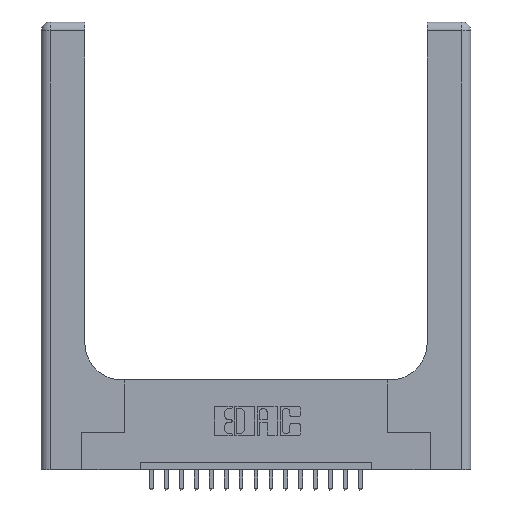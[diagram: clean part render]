
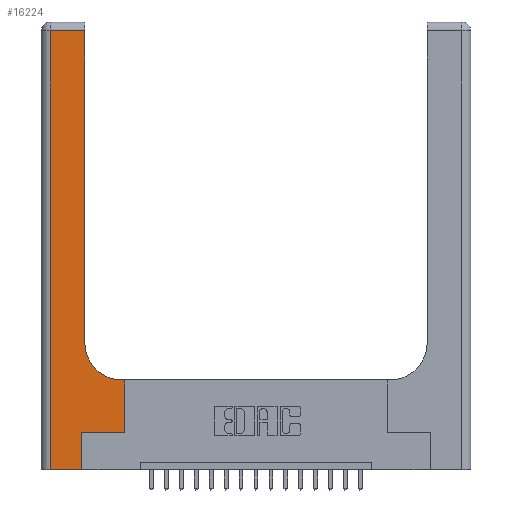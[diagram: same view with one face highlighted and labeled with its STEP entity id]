
A CAD part, top view. The second image highlights one B-rep face of the part: STEP entity #16224.
In plain terms, the highlighted planar face has unit normal (0, 0, 1).
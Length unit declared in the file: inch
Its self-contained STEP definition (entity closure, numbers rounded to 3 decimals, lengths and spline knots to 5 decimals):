
#102 = CARTESIAN_POINT ( 'NONE',  ( 0.2915, 2.94, 0.37 ) ) ;
#320 = ORIENTED_EDGE ( 'NONE', *, *, #8640, .T. ) ;
#1051 = EDGE_LOOP ( 'NONE', ( #19366, #9489, #320, #7773, #11748, #10143, #5590, #13464, #10118 ) ) ;
#1149 = CARTESIAN_POINT ( 'NONE',  ( 0.269, 0.25, 0.37 ) ) ;
#1548 = VECTOR ( 'NONE', #1977, 39.37008 ) ;
#1569 = DIRECTION ( 'NONE',  ( -1., 0., 0. ) ) ;
#1736 = LINE ( 'NONE', #12164, #11194 ) ;
#1977 = DIRECTION ( 'NONE',  ( 0., -1., 0. ) ) ;
#2047 = CARTESIAN_POINT ( 'NONE',  ( 0.269, 0., 0.37 ) ) ;
#2135 = EDGE_CURVE ( 'NONE', #11297, #3302, #1736, .T. ) ;
#2257 = CARTESIAN_POINT ( 'NONE',  ( 0.2915, 3., 0.37 ) ) ;
#2280 = EDGE_CURVE ( 'NONE', #13145, #3041, #5606, .T. ) ;
#2316 = CARTESIAN_POINT ( 'NONE',  ( 0.2915, 0.85, 0.37 ) ) ;
#2362 = DIRECTION ( 'NONE',  ( 0., 0., -1. ) ) ;
#2965 = VERTEX_POINT ( 'NONE', #15426 ) ;
#3041 = VERTEX_POINT ( 'NONE', #13840 ) ;
#3223 = VECTOR ( 'NONE', #8774, 39.37008 ) ;
#3302 = VERTEX_POINT ( 'NONE', #18086 ) ;
#3739 = LINE ( 'NONE', #2257, #8153 ) ;
#3854 = DIRECTION ( 'NONE',  ( 1., 0., 0. ) ) ;
#3926 = CARTESIAN_POINT ( 'NONE',  ( 0., 3., 0.37 ) ) ;
#4983 = LINE ( 'NONE', #10868, #19577 ) ;
#5110 = VECTOR ( 'NONE', #17660, 39.37008 ) ;
#5324 = CARTESIAN_POINT ( 'NONE',  ( 0.5585, 0.6, 0.37 ) ) ;
#5590 = ORIENTED_EDGE ( 'NONE', *, *, #14929, .T. ) ;
#5606 = LINE ( 'NONE', #8273, #5110 ) ;
#5673 = CARTESIAN_POINT ( 'NONE',  ( 0.269, 0., 0.37 ) ) ;
#5795 = CARTESIAN_POINT ( 'NONE',  ( 0., 0., 0.37 ) ) ;
#6699 = EDGE_CURVE ( 'NONE', #11780, #6821, #4983, .T. ) ;
#6821 = VERTEX_POINT ( 'NONE', #8727 ) ;
#7267 = EDGE_CURVE ( 'NONE', #2965, #15451, #16153, .T. ) ;
#7773 = ORIENTED_EDGE ( 'NONE', *, *, #7267, .T. ) ;
#8153 = VECTOR ( 'NONE', #14351, 39.37008 ) ;
#8273 = CARTESIAN_POINT ( 'NONE',  ( 0., 2.94, 0.37 ) ) ;
#8640 = EDGE_CURVE ( 'NONE', #3041, #2965, #18559, .T. ) ;
#8727 = CARTESIAN_POINT ( 'NONE',  ( 0.5415, 0.6, 0.37 ) ) ;
#8774 = DIRECTION ( 'NONE',  ( 0., 1., 0. ) ) ;
#9226 = LINE ( 'NONE', #5673, #13802 ) ;
#9489 = ORIENTED_EDGE ( 'NONE', *, *, #2280, .T. ) ;
#9979 = CARTESIAN_POINT ( 'NONE',  ( 0.06, 3., 0.37 ) ) ;
#10087 = DIRECTION ( 'NONE',  ( 0., 1., 0. ) ) ;
#10118 = ORIENTED_EDGE ( 'NONE', *, *, #12632, .T. ) ;
#10143 = ORIENTED_EDGE ( 'NONE', *, *, #2135, .T. ) ;
#10334 = AXIS2_PLACEMENT_3D ( 'NONE', #16062, #2362, #3854 ) ;
#10868 = CARTESIAN_POINT ( 'NONE',  ( 0.2915, 0.6, 0.37 ) ) ;
#11194 = VECTOR ( 'NONE', #13692, 39.37008 ) ;
#11297 = VERTEX_POINT ( 'NONE', #1149 ) ;
#11748 = ORIENTED_EDGE ( 'NONE', *, *, #16639, .T. ) ;
#11780 = VERTEX_POINT ( 'NONE', #5324 ) ;
#12164 = CARTESIAN_POINT ( 'NONE',  ( 0.269, 0.25, 0.37 ) ) ;
#12632 = EDGE_CURVE ( 'NONE', #6821, #13533, #15179, .T. ) ;
#12926 = LINE ( 'NONE', #13367, #3223 ) ;
#13091 = PLANE ( 'NONE',  #13895 ) ;
#13145 = VERTEX_POINT ( 'NONE', #102 ) ;
#13367 = CARTESIAN_POINT ( 'NONE',  ( 0.5585, 0.25, 0.37 ) ) ;
#13464 = ORIENTED_EDGE ( 'NONE', *, *, #6699, .T. ) ;
#13502 = EDGE_CURVE ( 'NONE', #13533, #13145, #3739, .T. ) ;
#13533 = VERTEX_POINT ( 'NONE', #2316 ) ;
#13584 = FACE_OUTER_BOUND ( 'NONE', #1051, .T. ) ;
#13692 = DIRECTION ( 'NONE',  ( 1., 0., 0. ) ) ;
#13802 = VECTOR ( 'NONE', #10087, 39.37008 ) ;
#13840 = CARTESIAN_POINT ( 'NONE',  ( 0.06, 2.94, 0.37 ) ) ;
#13895 = AXIS2_PLACEMENT_3D ( 'NONE', #3926, #17969, #16272 ) ;
#14351 = DIRECTION ( 'NONE',  ( 0., 1., 0. ) ) ;
#14682 = VECTOR ( 'NONE', #16629, 39.37008 ) ;
#14929 = EDGE_CURVE ( 'NONE', #3302, #11780, #12926, .T. ) ;
#15179 = CIRCLE ( 'NONE', #10334, 0.25 ) ;
#15426 = CARTESIAN_POINT ( 'NONE',  ( 0.06, 0., 0.37 ) ) ;
#15451 = VERTEX_POINT ( 'NONE', #2047 ) ;
#16062 = CARTESIAN_POINT ( 'NONE',  ( 0.5415, 0.85, 0.37 ) ) ;
#16153 = LINE ( 'NONE', #5795, #14682 ) ;
#16224 = ADVANCED_FACE ( 'NONE', ( #13584 ), #13091, .F. ) ;
#16272 = DIRECTION ( 'NONE',  ( -1., 0., 0. ) ) ;
#16629 = DIRECTION ( 'NONE',  ( 1., 0., 0. ) ) ;
#16639 = EDGE_CURVE ( 'NONE', #15451, #11297, #9226, .T. ) ;
#17660 = DIRECTION ( 'NONE',  ( -1., 0., 0. ) ) ;
#17969 = DIRECTION ( 'NONE',  ( 0., 0., -1. ) ) ;
#18086 = CARTESIAN_POINT ( 'NONE',  ( 0.5585, 0.25, 0.37 ) ) ;
#18559 = LINE ( 'NONE', #9979, #1548 ) ;
#19366 = ORIENTED_EDGE ( 'NONE', *, *, #13502, .T. ) ;
#19577 = VECTOR ( 'NONE', #1569, 39.37008 ) ;
